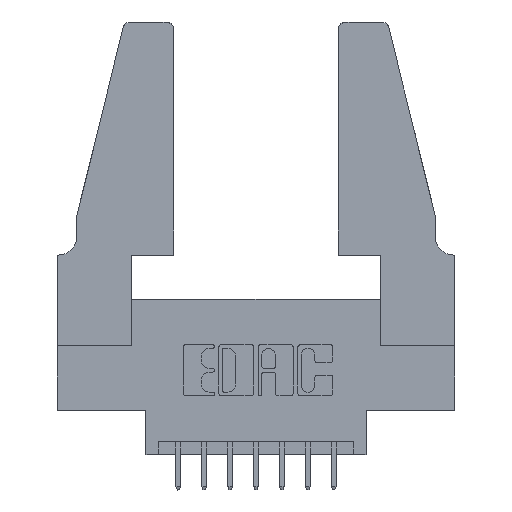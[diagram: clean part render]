
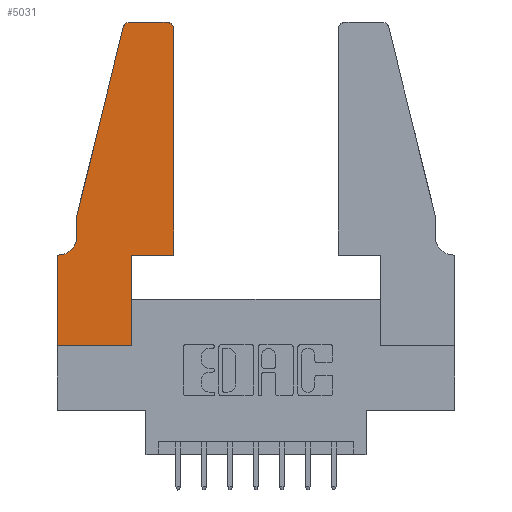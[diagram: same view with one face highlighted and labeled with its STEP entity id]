
A CAD part, top view. The second image highlights one B-rep face of the part: STEP entity #5031.
In plain terms, the highlighted planar face has unit normal (0, 0, 1).
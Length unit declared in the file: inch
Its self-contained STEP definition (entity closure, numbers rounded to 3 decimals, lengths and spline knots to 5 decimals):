
#638 = CARTESIAN_POINT ( 'NONE',  ( 0.0755, 0.42, 0.37 ) ) ;
#796 = DIRECTION ( 'NONE',  ( 0., 0., 1. ) ) ;
#958 = ORIENTED_EDGE ( 'NONE', *, *, #10109, .T. ) ;
#990 = CARTESIAN_POINT ( 'NONE',  ( 0.0755, 0.5, 0.37 ) ) ;
#1050 = CARTESIAN_POINT ( 'NONE',  ( 0.4205, 1.25, 0.37 ) ) ;
#1093 = CARTESIAN_POINT ( 'NONE',  ( 0.0755, 0.5, 0.37 ) ) ;
#1153 = DIRECTION ( 'NONE',  ( 0., -1., 0. ) ) ;
#1179 = LINE ( 'NONE', #990, #11974 ) ;
#1404 = ORIENTED_EDGE ( 'NONE', *, *, #5559, .T. ) ;
#1683 = CARTESIAN_POINT ( 'NONE',  ( 0.0755, 0.35, 0.37 ) ) ;
#1685 = LINE ( 'NONE', #9072, #8542 ) ;
#1742 = CARTESIAN_POINT ( 'NONE',  ( 0.2605, 1.25, 0.37 ) ) ;
#1749 = DIRECTION ( 'NONE',  ( -0.239, -0.971, 0. ) ) ;
#1761 = VECTOR ( 'NONE', #7489, 39.37008 ) ;
#1787 = VECTOR ( 'NONE', #7743, 39.37008 ) ;
#2044 = ORIENTED_EDGE ( 'NONE', *, *, #9961, .T. ) ;
#2062 = CARTESIAN_POINT ( 'NONE',  ( 0., 0., 0.37 ) ) ;
#2093 = DIRECTION ( 'NONE',  ( 0., 0., 1. ) ) ;
#2282 = DIRECTION ( 'NONE',  ( 0., 0., 1. ) ) ;
#2320 = ORIENTED_EDGE ( 'NONE', *, *, #2978, .T. ) ;
#2367 = CIRCLE ( 'NONE', #9491, 0.03 ) ;
#2476 = ORIENTED_EDGE ( 'NONE', *, *, #5176, .T. ) ;
#2610 = CARTESIAN_POINT ( 'NONE',  ( 0., 0., 0.37 ) ) ;
#2635 = LINE ( 'NONE', #1683, #6900 ) ;
#2818 = DIRECTION ( 'NONE',  ( 0., 0., -1. ) ) ;
#2978 = EDGE_CURVE ( 'NONE', #10054, #9161, #2367, .T. ) ;
#3027 = PLANE ( 'NONE',  #9821 ) ;
#3356 = EDGE_CURVE ( 'NONE', #9837, #11767, #8613, .T. ) ;
#3458 = CARTESIAN_POINT ( 'NONE',  ( 0.284, 1.25, 0.37 ) ) ;
#3552 = VERTEX_POINT ( 'NONE', #8988 ) ;
#3783 = AXIS2_PLACEMENT_3D ( 'NONE', #7122, #2282, #11881 ) ;
#3900 = VERTEX_POINT ( 'NONE', #11967 ) ;
#3966 = ORIENTED_EDGE ( 'NONE', *, *, #8548, .T. ) ;
#4574 = CARTESIAN_POINT ( 'NONE',  ( 0.0755, 0.5, 0.37 ) ) ;
#4712 = CARTESIAN_POINT ( 'NONE',  ( 0., 0., 0.37 ) ) ;
#4841 = DIRECTION ( 'NONE',  ( 0., -1., 0. ) ) ;
#4929 = VERTEX_POINT ( 'NONE', #2610 ) ;
#5031 = ADVANCED_FACE ( 'NONE', ( #7983 ), #3027, .T. ) ;
#5176 = EDGE_CURVE ( 'NONE', #4929, #3552, #5507, .T. ) ;
#5220 = CARTESIAN_POINT ( 'NONE',  ( 0.2865, 0.35, 0.37 ) ) ;
#5507 = LINE ( 'NONE', #4712, #1761 ) ;
#5546 = CARTESIAN_POINT ( 'NONE',  ( 0.0055, 0.35, 0.37 ) ) ;
#5559 = EDGE_CURVE ( 'NONE', #3900, #4929, #5797, .T. ) ;
#5602 = DIRECTION ( 'NONE',  ( -1., 0., 0. ) ) ;
#5797 = LINE ( 'NONE', #2062, #6441 ) ;
#5995 = VERTEX_POINT ( 'NONE', #638 ) ;
#6074 = CARTESIAN_POINT ( 'NONE',  ( 0.25487, 1.22718, 0.37 ) ) ;
#6078 = DIRECTION ( 'NONE',  ( 0., 1., 0. ) ) ;
#6441 = VECTOR ( 'NONE', #1153, 39.37008 ) ;
#6508 = DIRECTION ( 'NONE',  ( -1., 0., 0. ) ) ;
#6591 = DIRECTION ( 'NONE',  ( -1., 0., 0. ) ) ;
#6655 = EDGE_LOOP ( 'NONE', ( #9631, #3966, #10251, #2044, #7273, #958, #1404, #2476, #12279, #11670, #6940, #2320 ) ) ;
#6806 = EDGE_CURVE ( 'NONE', #3552, #8066, #8637, .T. ) ;
#6881 = VECTOR ( 'NONE', #6078, 39.37008 ) ;
#6900 = VECTOR ( 'NONE', #6508, 39.37008 ) ;
#6924 = CARTESIAN_POINT ( 'NONE',  ( 0., 0.35, 0.37 ) ) ;
#6926 = CARTESIAN_POINT ( 'NONE',  ( 0.2865, 0.35, 0.37 ) ) ;
#6940 = ORIENTED_EDGE ( 'NONE', *, *, #9125, .T. ) ;
#7081 = EDGE_CURVE ( 'NONE', #5995, #7124, #8693, .T. ) ;
#7122 = CARTESIAN_POINT ( 'NONE',  ( 0.284, 1.22, 0.37 ) ) ;
#7124 = VERTEX_POINT ( 'NONE', #5546 ) ;
#7126 = VECTOR ( 'NONE', #5602, 39.37008 ) ;
#7273 = ORIENTED_EDGE ( 'NONE', *, *, #7081, .T. ) ;
#7489 = DIRECTION ( 'NONE',  ( 1., 0., 0. ) ) ;
#7742 = DIRECTION ( 'NONE',  ( 1., 0., 0. ) ) ;
#7743 = DIRECTION ( 'NONE',  ( 0., 1., 0. ) ) ;
#7970 = LINE ( 'NONE', #10036, #6881 ) ;
#7983 = FACE_OUTER_BOUND ( 'NONE', #6655, .T. ) ;
#8066 = VERTEX_POINT ( 'NONE', #5220 ) ;
#8184 = VERTEX_POINT ( 'NONE', #3458 ) ;
#8542 = VECTOR ( 'NONE', #10929, 39.37008 ) ;
#8548 = EDGE_CURVE ( 'NONE', #8184, #9837, #9921, .T. ) ;
#8613 = LINE ( 'NONE', #4574, #8771 ) ;
#8637 = LINE ( 'NONE', #6926, #1787 ) ;
#8693 = CIRCLE ( 'NONE', #12530, 0.07 ) ;
#8771 = VECTOR ( 'NONE', #1749, 39.37008 ) ;
#8988 = CARTESIAN_POINT ( 'NONE',  ( 0.2865, 0., 0.37 ) ) ;
#9072 = CARTESIAN_POINT ( 'NONE',  ( 0.4505, 0.35, 0.37 ) ) ;
#9125 = EDGE_CURVE ( 'NONE', #9253, #10054, #7970, .T. ) ;
#9161 = VERTEX_POINT ( 'NONE', #1050 ) ;
#9217 = CARTESIAN_POINT ( 'NONE',  ( 0.0055, 0.42, 0.37 ) ) ;
#9253 = VERTEX_POINT ( 'NONE', #11736 ) ;
#9491 = AXIS2_PLACEMENT_3D ( 'NONE', #12502, #796, #11609 ) ;
#9631 = ORIENTED_EDGE ( 'NONE', *, *, #11660, .T. ) ;
#9821 = AXIS2_PLACEMENT_3D ( 'NONE', #6924, #2093, #7742 ) ;
#9837 = VERTEX_POINT ( 'NONE', #6074 ) ;
#9921 = CIRCLE ( 'NONE', #3783, 0.03 ) ;
#9961 = EDGE_CURVE ( 'NONE', #11767, #5995, #1179, .T. ) ;
#10036 = CARTESIAN_POINT ( 'NONE',  ( 0.4505, 0.35, 0.37 ) ) ;
#10054 = VERTEX_POINT ( 'NONE', #11352 ) ;
#10109 = EDGE_CURVE ( 'NONE', #7124, #3900, #2635, .T. ) ;
#10251 = ORIENTED_EDGE ( 'NONE', *, *, #3356, .T. ) ;
#10929 = DIRECTION ( 'NONE',  ( 1., 0., 0. ) ) ;
#11352 = CARTESIAN_POINT ( 'NONE',  ( 0.4505, 1.22, 0.37 ) ) ;
#11479 = EDGE_CURVE ( 'NONE', #8066, #9253, #1685, .T. ) ;
#11609 = DIRECTION ( 'NONE',  ( 1., 0., 0. ) ) ;
#11660 = EDGE_CURVE ( 'NONE', #9161, #8184, #12437, .T. ) ;
#11670 = ORIENTED_EDGE ( 'NONE', *, *, #11479, .T. ) ;
#11736 = CARTESIAN_POINT ( 'NONE',  ( 0.4505, 0.35, 0.37 ) ) ;
#11767 = VERTEX_POINT ( 'NONE', #1093 ) ;
#11881 = DIRECTION ( 'NONE',  ( 1., 0., 0. ) ) ;
#11967 = CARTESIAN_POINT ( 'NONE',  ( 0., 0.35, 0.37 ) ) ;
#11974 = VECTOR ( 'NONE', #4841, 39.37008 ) ;
#12279 = ORIENTED_EDGE ( 'NONE', *, *, #6806, .T. ) ;
#12437 = LINE ( 'NONE', #1742, #7126 ) ;
#12502 = CARTESIAN_POINT ( 'NONE',  ( 0.4205, 1.22, 0.37 ) ) ;
#12530 = AXIS2_PLACEMENT_3D ( 'NONE', #9217, #2818, #6591 ) ;
